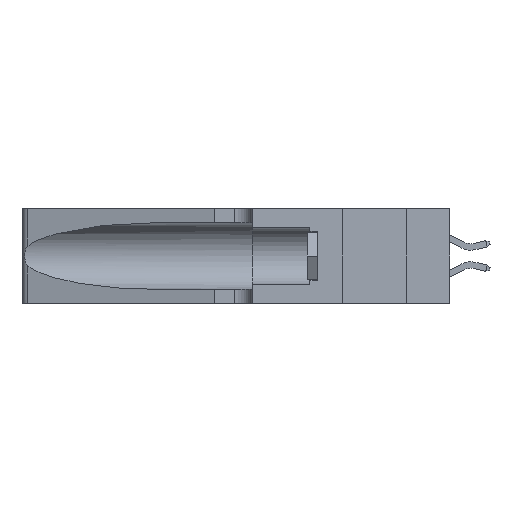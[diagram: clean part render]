
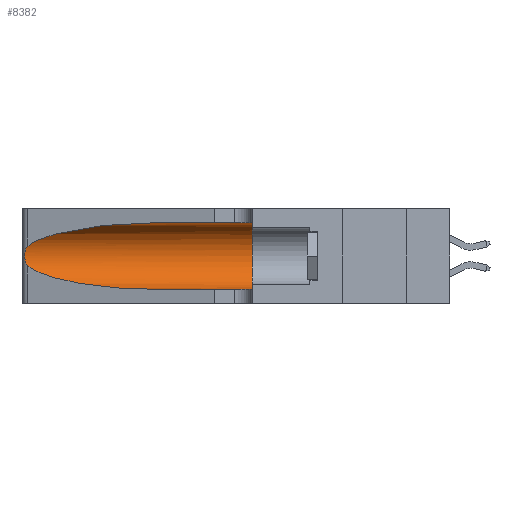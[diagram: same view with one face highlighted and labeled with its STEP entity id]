
A CAD part, left-side view. The second image highlights one B-rep face of the part: STEP entity #8382.
In plain terms, the highlighted cylindrical face has radius 3.308 mm (diameter 6.617 mm), a partial arc.
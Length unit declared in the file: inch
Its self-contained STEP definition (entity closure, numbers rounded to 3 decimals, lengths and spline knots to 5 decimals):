
#85 = CARTESIAN_POINT ( 'NONE',  ( 0.18966, 0.96281, 0.05475 ) ) ;
#124 =( BOUNDED_CURVE ( )  B_SPLINE_CURVE ( 3, ( #2044, #20338, #85, #13220 ),
 .UNSPECIFIED., .F., .T. ) 
 B_SPLINE_CURVE_WITH_KNOTS ( ( 4, 4 ),
 ( 3.44316, 4.71239 ),
 .UNSPECIFIED. ) 
 CURVE ( )  GEOMETRIC_REPRESENTATION_ITEM ( )  RATIONAL_B_SPLINE_CURVE ( ( 1., 0.87, 0.87, 1. ) ) 
 REPRESENTATION_ITEM ( '' )  );
#395 = CARTESIAN_POINT ( 'NONE',  ( 0.25487, 1.22718, 0.14631 ) ) ;
#510 = CARTESIAN_POINT ( 'NONE',  ( 0.25854, 1.2359, 0.20912 ) ) ;
#1674 = VERTEX_POINT ( 'NONE', #395 ) ;
#2044 = CARTESIAN_POINT ( 'NONE',  ( 0.25487, 1.22718, 0.14631 ) ) ;
#2129 = CIRCLE ( 'NONE', #21600, 0.13025 ) ;
#2522 = CARTESIAN_POINT ( 'NONE',  ( 0.26075, 1.23896, 0.19203 ) ) ;
#2594 = VECTOR ( 'NONE', #22945, 39.37008 ) ;
#3037 = ORIENTED_EDGE ( 'NONE', *, *, #11962, .F. ) ;
#3285 = VERTEX_POINT ( 'NONE', #6365 ) ;
#3401 = VERTEX_POINT ( 'NONE', #10290 ) ;
#4441 = CARTESIAN_POINT ( 'NONE',  ( 0.26017, 1.23833, 0.17102 ) ) ;
#5266 = CARTESIAN_POINT ( 'NONE',  ( 0.1305, 0.72297, 0.31525 ) ) ;
#5346 = CARTESIAN_POINT ( 'NONE',  ( 0.2373, 1.15595, 0.28018 ) ) ;
#6309 = CARTESIAN_POINT ( 'NONE',  ( 0.25789, 1.23486, 0.15765 ) ) ;
#6365 = CARTESIAN_POINT ( 'NONE',  ( 0.1305, 0.72297, 0.31525 ) ) ;
#6568 = VERTEX_POINT ( 'NONE', #6581 ) ;
#6581 = CARTESIAN_POINT ( 'NONE',  ( 0.1305, 0.35, 0.31525 ) ) ;
#6665 = DIRECTION ( 'NONE',  ( 0., -1., 0. ) ) ;
#6741 = CARTESIAN_POINT ( 'NONE',  ( 0.1305, 1.61858, 0.185 ) ) ;
#7621 = EDGE_CURVE ( 'NONE', #6568, #7809, #2129, .T. ) ;
#7809 = VERTEX_POINT ( 'NONE', #13937 ) ;
#7867 = ORIENTED_EDGE ( 'NONE', *, *, #7621, .F. ) ;
#7890 = CARTESIAN_POINT ( 'NONE',  ( 0.1305, 0.35, 0.185 ) ) ;
#8077 = CARTESIAN_POINT ( 'NONE',  ( 0.25487, 1.22718, 0.22369 ) ) ;
#8164 = CARTESIAN_POINT ( 'NONE',  ( 0.25555, 1.22993, 0.14849 ) ) ;
#8382 = ADVANCED_FACE ( 'NONE', ( #9401 ), #8814, .F. ) ;
#8814 = CYLINDRICAL_SURFACE ( 'NONE', #16657, 0.13025 ) ;
#9401 = FACE_OUTER_BOUND ( 'NONE', #18067, .T. ) ;
#9740 = DIRECTION ( 'NONE',  ( 0., 0., 1. ) ) ;
#9931 = CARTESIAN_POINT ( 'NONE',  ( 0.25555, 1.22994, 0.2215 ) ) ;
#10290 = CARTESIAN_POINT ( 'NONE',  ( 0.1305, 0.72297, 0.05475 ) ) ;
#10818 = CARTESIAN_POINT ( 'NONE',  ( 0.18966, 0.96281, 0.31525 ) ) ;
#11301 = VERTEX_POINT ( 'NONE', #14406 ) ;
#11517 = EDGE_CURVE ( 'NONE', #1674, #3401, #124, .T. ) ;
#11547 = VECTOR ( 'NONE', #21741, 39.37008 ) ;
#11769 = CARTESIAN_POINT ( 'NONE',  ( 0.25787, 1.23484, 0.2124 ) ) ;
#11962 = EDGE_CURVE ( 'NONE', #3285, #6568, #12105, .T. ) ;
#12105 = LINE ( 'NONE', #23458, #11547 ) ;
#13220 = CARTESIAN_POINT ( 'NONE',  ( 0.1305, 0.72297, 0.05475 ) ) ;
#13599 = CARTESIAN_POINT ( 'NONE',  ( 0.26018, 1.23835, 0.19895 ) ) ;
#13937 = CARTESIAN_POINT ( 'NONE',  ( 0.1305, 0.35, 0.05475 ) ) ;
#14249 = EDGE_CURVE ( 'NONE', #3401, #7809, #17217, .T. ) ;
#14406 = CARTESIAN_POINT ( 'NONE',  ( 0.25487, 1.22718, 0.22369 ) ) ;
#15395 = CARTESIAN_POINT ( 'NONE',  ( 0.26075, 1.23896, 0.178 ) ) ;
#15554 = ORIENTED_EDGE ( 'NONE', *, *, #14249, .T. ) ;
#16657 = AXIS2_PLACEMENT_3D ( 'NONE', #6741, #6665, #19314 ) ;
#17186 = CARTESIAN_POINT ( 'NONE',  ( 0.25856, 1.23593, 0.16098 ) ) ;
#17217 = LINE ( 'NONE', #21142, #2594 ) ;
#18050 = CARTESIAN_POINT ( 'NONE',  ( 0.25487, 1.22718, 0.22369 ) ) ;
#18067 = EDGE_LOOP ( 'NONE', ( #21836, #19164, #20569, #15554, #7867, #3037 ) ) ;
#18950 =( BOUNDED_CURVE ( )  B_SPLINE_CURVE ( 3, ( #5266, #10818, #5346, #18050 ),
 .UNSPECIFIED., .F., .F. ) 
 B_SPLINE_CURVE_WITH_KNOTS ( ( 4, 4 ),
 ( 1.5708, 2.84003 ),
 .UNSPECIFIED. ) 
 CURVE ( )  GEOMETRIC_REPRESENTATION_ITEM ( )  RATIONAL_B_SPLINE_CURVE ( ( 1., 0.87, 0.87, 1. ) ) 
 REPRESENTATION_ITEM ( '' )  );
#18973 = CARTESIAN_POINT ( 'NONE',  ( 0.25639, 1.23186, 0.15144 ) ) ;
#19164 = ORIENTED_EDGE ( 'NONE', *, *, #20621, .T. ) ;
#19314 = DIRECTION ( 'NONE',  ( 0., 0., -1. ) ) ;
#20338 = CARTESIAN_POINT ( 'NONE',  ( 0.2373, 1.15595, 0.08982 ) ) ;
#20524 = DIRECTION ( 'NONE',  ( 0., 1., 0. ) ) ;
#20569 = ORIENTED_EDGE ( 'NONE', *, *, #11517, .T. ) ;
#20621 = EDGE_CURVE ( 'NONE', #11301, #1674, #23141, .T. ) ;
#20786 = CARTESIAN_POINT ( 'NONE',  ( 0.25487, 1.22718, 0.14631 ) ) ;
#21142 = CARTESIAN_POINT ( 'NONE',  ( 0.1305, 1.61858, 0.05475 ) ) ;
#21600 = AXIS2_PLACEMENT_3D ( 'NONE', #7890, #20524, #9740 ) ;
#21741 = DIRECTION ( 'NONE',  ( 0., -1., 0. ) ) ;
#21836 = ORIENTED_EDGE ( 'NONE', *, *, #22778, .T. ) ;
#22518 = CARTESIAN_POINT ( 'NONE',  ( 0.25639, 1.23184, 0.21858 ) ) ;
#22778 = EDGE_CURVE ( 'NONE', #3285, #11301, #18950, .T. ) ;
#22945 = DIRECTION ( 'NONE',  ( 0., -1., 0. ) ) ;
#23141 = B_SPLINE_CURVE_WITH_KNOTS ( 'NONE', 3,
 ( #8077, #9931, #22518, #11769, #510, #13599, #2522, #15395, #4441, #17186, #6309, #18973, #8164, #20786 ),
 .UNSPECIFIED., .F., .F.,
 ( 4, 2, 2, 2, 2, 2, 4 ),
 ( 0., 0.00027, 0.00053, 0.00107, 0.0016, 0.00187, 0.00214 ),
 .UNSPECIFIED. ) ;
#23458 = CARTESIAN_POINT ( 'NONE',  ( 0.1305, 1.61858, 0.31525 ) ) ;
